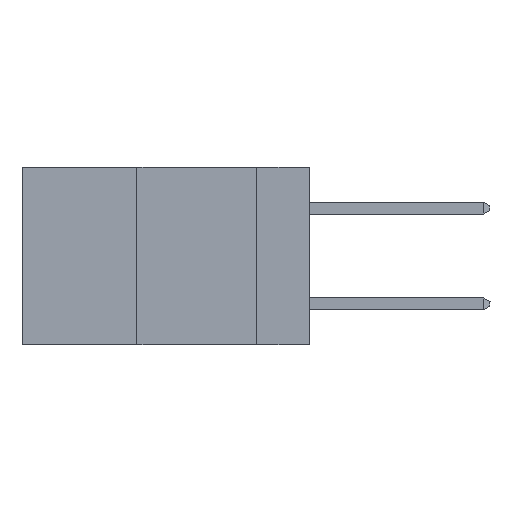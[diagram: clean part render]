
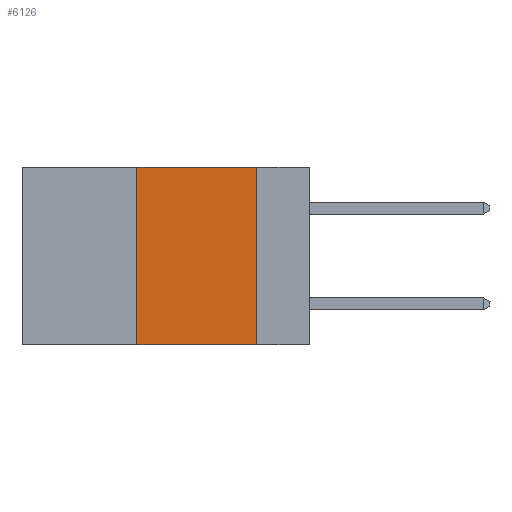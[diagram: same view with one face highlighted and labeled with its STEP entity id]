
A CAD part, left-side view. The second image highlights one B-rep face of the part: STEP entity #6126.
In plain terms, the highlighted planar face has unit normal (-1, 0, 0).
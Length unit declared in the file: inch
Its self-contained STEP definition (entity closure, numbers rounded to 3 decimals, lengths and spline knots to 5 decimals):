
#112 = EDGE_LOOP ( 'NONE', ( #6242, #7696, #11555, #4989 ) ) ;
#653 = EDGE_CURVE ( 'NONE', #7230, #7697, #4167, .T. ) ;
#709 = CARTESIAN_POINT ( 'NONE',  ( 0., 0.6, 0. ) ) ;
#1253 = AXIS2_PLACEMENT_3D ( 'NONE', #709, #11665, #2413 ) ;
#1849 = CARTESIAN_POINT ( 'NONE',  ( 0., 0.6, 0. ) ) ;
#1970 = EDGE_CURVE ( 'NONE', #5324, #7230, #5809, .T. ) ;
#2358 = CARTESIAN_POINT ( 'NONE',  ( 0., 0.11, 0. ) ) ;
#2413 = DIRECTION ( 'NONE',  ( 0., 0., -1. ) ) ;
#2518 = DIRECTION ( 'NONE',  ( 0., 0., -1. ) ) ;
#2550 = VECTOR ( 'NONE', #9096, 39.37008 ) ;
#3014 = DIRECTION ( 'NONE',  ( 0., -1., 0. ) ) ;
#3687 = CARTESIAN_POINT ( 'NONE',  ( 0., 0.36, 0. ) ) ;
#3975 = CARTESIAN_POINT ( 'NONE',  ( 0., 0.36, -0.37 ) ) ;
#4091 = VECTOR ( 'NONE', #3014, 39.37008 ) ;
#4167 = LINE ( 'NONE', #11652, #5610 ) ;
#4989 = ORIENTED_EDGE ( 'NONE', *, *, #10685, .T. ) ;
#5287 = VECTOR ( 'NONE', #9587, 39.37008 ) ;
#5324 = VERTEX_POINT ( 'NONE', #8556 ) ;
#5584 = LINE ( 'NONE', #3687, #2550 ) ;
#5610 = VECTOR ( 'NONE', #2518, 39.37008 ) ;
#5809 = LINE ( 'NONE', #1849, #4091 ) ;
#6126 = ADVANCED_FACE ( 'NONE', ( #10801 ), #10908, .F. ) ;
#6242 = ORIENTED_EDGE ( 'NONE', *, *, #653, .F. ) ;
#6488 = VERTEX_POINT ( 'NONE', #3975 ) ;
#6826 = CARTESIAN_POINT ( 'NONE',  ( 0., 0.6, -0.37 ) ) ;
#7230 = VERTEX_POINT ( 'NONE', #2358 ) ;
#7696 = ORIENTED_EDGE ( 'NONE', *, *, #1970, .F. ) ;
#7697 = VERTEX_POINT ( 'NONE', #8709 ) ;
#8556 = CARTESIAN_POINT ( 'NONE',  ( 0., 0.36, 0. ) ) ;
#8709 = CARTESIAN_POINT ( 'NONE',  ( 0., 0.11, -0.37 ) ) ;
#9096 = DIRECTION ( 'NONE',  ( 0., 0., 1. ) ) ;
#9461 = LINE ( 'NONE', #6826, #5287 ) ;
#9587 = DIRECTION ( 'NONE',  ( 0., -1., 0. ) ) ;
#10576 = EDGE_CURVE ( 'NONE', #6488, #5324, #5584, .T. ) ;
#10685 = EDGE_CURVE ( 'NONE', #6488, #7697, #9461, .T. ) ;
#10801 = FACE_OUTER_BOUND ( 'NONE', #112, .T. ) ;
#10908 = PLANE ( 'NONE',  #1253 ) ;
#11555 = ORIENTED_EDGE ( 'NONE', *, *, #10576, .F. ) ;
#11652 = CARTESIAN_POINT ( 'NONE',  ( 0., 0.11, 0. ) ) ;
#11665 = DIRECTION ( 'NONE',  ( 1., 0., 0. ) ) ;
